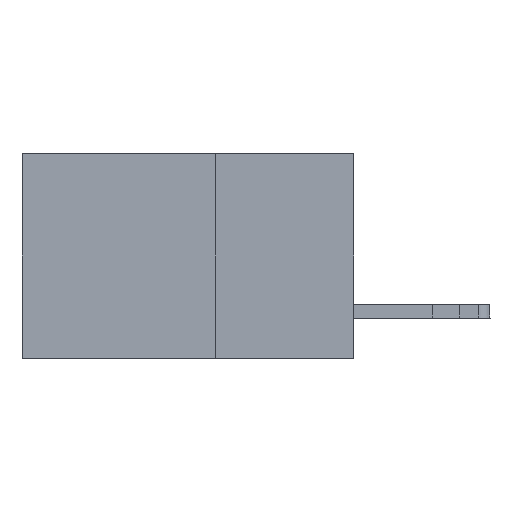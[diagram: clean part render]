
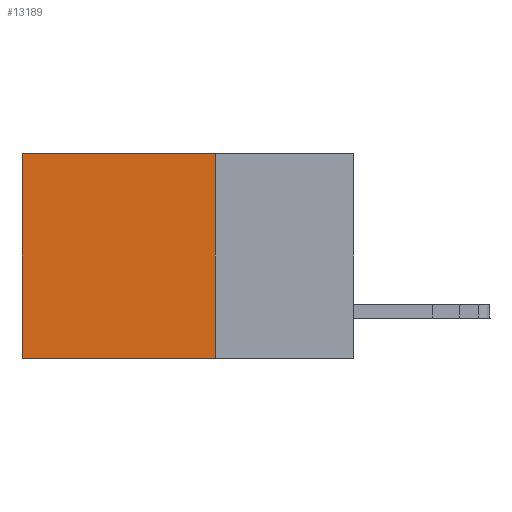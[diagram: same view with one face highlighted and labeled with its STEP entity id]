
A CAD part, left-side view. The second image highlights one B-rep face of the part: STEP entity #13189.
In plain terms, the highlighted planar face has unit normal (-1, 0, 0).
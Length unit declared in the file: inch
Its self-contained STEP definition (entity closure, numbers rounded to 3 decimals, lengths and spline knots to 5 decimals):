
#25 = VERTEX_POINT ( 'NONE', #12877 ) ;
#401 = ORIENTED_EDGE ( 'NONE', *, *, #4073, .F. ) ;
#479 = VERTEX_POINT ( 'NONE', #2416 ) ;
#884 = CARTESIAN_POINT ( 'NONE',  ( 0.2875, 0.25, 0. ) ) ;
#1725 = DIRECTION ( 'NONE',  ( 0., 0., -1. ) ) ;
#1999 = ORIENTED_EDGE ( 'NONE', *, *, #13378, .T. ) ;
#2416 = CARTESIAN_POINT ( 'NONE',  ( 0.2875, 0.25, 0. ) ) ;
#4073 = EDGE_CURVE ( 'NONE', #479, #27363, #36415, .T. ) ;
#5714 = VERTEX_POINT ( 'NONE', #9788 ) ;
#6863 = DIRECTION ( 'NONE',  ( 0., 0., -1. ) ) ;
#8611 = VECTOR ( 'NONE', #6863, 39.37008 ) ;
#9467 = LINE ( 'NONE', #9889, #33757 ) ;
#9788 = CARTESIAN_POINT ( 'NONE',  ( 0.2875, 0.6, 0. ) ) ;
#9889 = CARTESIAN_POINT ( 'NONE',  ( 0.2875, 0.25, -0.37 ) ) ;
#12215 = LINE ( 'NONE', #884, #26574 ) ;
#12676 = CARTESIAN_POINT ( 'NONE',  ( 0.2875, 0.25, 0. ) ) ;
#12877 = CARTESIAN_POINT ( 'NONE',  ( 0.2875, 0.6, -0.37 ) ) ;
#12901 = DIRECTION ( 'NONE',  ( 0., 1., 0. ) ) ;
#13009 = CARTESIAN_POINT ( 'NONE',  ( 0.2875, 0.6, 0. ) ) ;
#13055 = PLANE ( 'NONE',  #25130 ) ;
#13099 = EDGE_CURVE ( 'NONE', #5714, #25, #24869, .T. ) ;
#13189 = ADVANCED_FACE ( 'NONE', ( #27534 ), #13055, .F. ) ;
#13378 = EDGE_CURVE ( 'NONE', #479, #5714, #12215, .T. ) ;
#14007 = EDGE_CURVE ( 'NONE', #27363, #25, #9467, .T. ) ;
#15676 = CARTESIAN_POINT ( 'NONE',  ( 0.2875, 0.25, 0. ) ) ;
#17212 = VECTOR ( 'NONE', #1725, 39.37008 ) ;
#17485 = DIRECTION ( 'NONE',  ( 1., 0., 0. ) ) ;
#17935 = EDGE_LOOP ( 'NONE', ( #29741, #36481, #401, #1999 ) ) ;
#23364 = DIRECTION ( 'NONE',  ( 0., 1., 0. ) ) ;
#24869 = LINE ( 'NONE', #13009, #17212 ) ;
#25130 = AXIS2_PLACEMENT_3D ( 'NONE', #12676, #17485, #32278 ) ;
#26574 = VECTOR ( 'NONE', #23364, 39.37008 ) ;
#27363 = VERTEX_POINT ( 'NONE', #30145 ) ;
#27534 = FACE_OUTER_BOUND ( 'NONE', #17935, .T. ) ;
#29741 = ORIENTED_EDGE ( 'NONE', *, *, #13099, .T. ) ;
#30145 = CARTESIAN_POINT ( 'NONE',  ( 0.2875, 0.25, -0.37 ) ) ;
#32278 = DIRECTION ( 'NONE',  ( 0., 0., -1. ) ) ;
#33757 = VECTOR ( 'NONE', #12901, 39.37008 ) ;
#36415 = LINE ( 'NONE', #15676, #8611 ) ;
#36481 = ORIENTED_EDGE ( 'NONE', *, *, #14007, .F. ) ;
